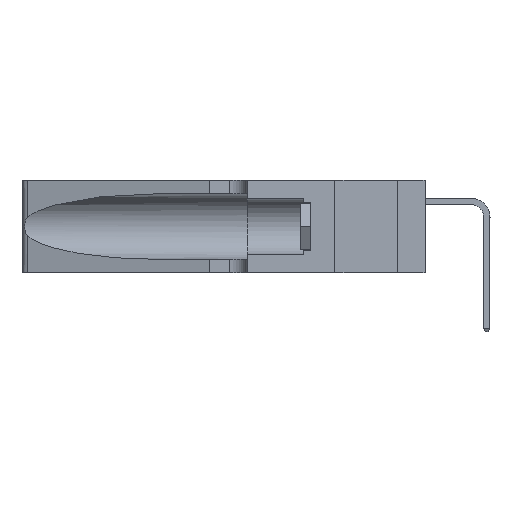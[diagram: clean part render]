
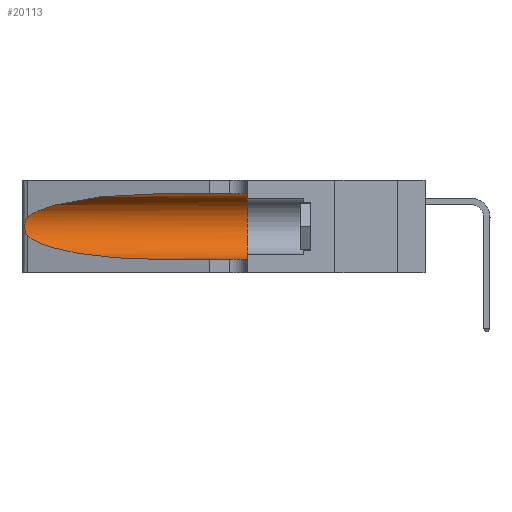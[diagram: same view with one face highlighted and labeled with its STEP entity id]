
A CAD part, left-side view. The second image highlights one B-rep face of the part: STEP entity #20113.
In plain terms, the highlighted cylindrical face has radius 3.308 mm (diameter 6.617 mm), a partial arc.
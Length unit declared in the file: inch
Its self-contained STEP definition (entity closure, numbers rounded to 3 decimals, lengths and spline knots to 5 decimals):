
#367 = B_SPLINE_CURVE_WITH_KNOTS ( 'NONE', 3,
 ( #2973, #14654, #8839, #22575, #10785, #24509, #12739, #1071, #14736, #3061, #16752, #5017, #18703, #6977 ),
 .UNSPECIFIED., .F., .F.,
 ( 4, 2, 2, 2, 2, 2, 4 ),
 ( 0., 0.00027, 0.00053, 0.00107, 0.0016, 0.00187, 0.00214 ),
 .UNSPECIFIED. ) ;
#808 = CARTESIAN_POINT ( 'NONE',  ( 0.25487, 1.22718, 0.14631 ) ) ;
#1071 = CARTESIAN_POINT ( 'NONE',  ( 0.26075, 1.23896, 0.178 ) ) ;
#1658 = VERTEX_POINT ( 'NONE', #12820 ) ;
#1889 = EDGE_CURVE ( 'NONE', #17701, #10730, #15651, .T. ) ;
#2789 = CARTESIAN_POINT ( 'NONE',  ( 0.1305, 0.72297, 0.31525 ) ) ;
#2973 = CARTESIAN_POINT ( 'NONE',  ( 0.25487, 1.22718, 0.22369 ) ) ;
#3061 = CARTESIAN_POINT ( 'NONE',  ( 0.25856, 1.23593, 0.16098 ) ) ;
#3597 = AXIS2_PLACEMENT_3D ( 'NONE', #19043, #22995, #11213 ) ;
#3985 = DIRECTION ( 'NONE',  ( 0., -1., 0. ) ) ;
#4210 = ORIENTED_EDGE ( 'NONE', *, *, #18114, .T. ) ;
#4444 = VECTOR ( 'NONE', #5754, 39.37008 ) ;
#4894 = EDGE_CURVE ( 'NONE', #23145, #14350, #22512, .T. ) ;
#5017 = CARTESIAN_POINT ( 'NONE',  ( 0.25639, 1.23186, 0.15144 ) ) ;
#5339 = VERTEX_POINT ( 'NONE', #7883 ) ;
#5754 = DIRECTION ( 'NONE',  ( 0., -1., 0. ) ) ;
#5861 = DIRECTION ( 'NONE',  ( 0., 1., 0. ) ) ;
#5895 = ORIENTED_EDGE ( 'NONE', *, *, #16063, .F. ) ;
#6423 = CARTESIAN_POINT ( 'NONE',  ( 0.1305, 0.72297, 0.05475 ) ) ;
#6775 = CARTESIAN_POINT ( 'NONE',  ( 0.1305, 0.35, 0.05475 ) ) ;
#6977 = CARTESIAN_POINT ( 'NONE',  ( 0.25487, 1.22718, 0.14631 ) ) ;
#7883 = CARTESIAN_POINT ( 'NONE',  ( 0.25487, 1.22718, 0.22369 ) ) ;
#8573 = CARTESIAN_POINT ( 'NONE',  ( 0.2373, 1.15595, 0.08982 ) ) ;
#8663 = CARTESIAN_POINT ( 'NONE',  ( 0.2373, 1.15595, 0.28018 ) ) ;
#8712 = CARTESIAN_POINT ( 'NONE',  ( 0.1305, 0.35, 0.31525 ) ) ;
#8839 = CARTESIAN_POINT ( 'NONE',  ( 0.25639, 1.23184, 0.21858 ) ) ;
#9137 = LINE ( 'NONE', #19554, #23550 ) ;
#10332 = CARTESIAN_POINT ( 'NONE',  ( 0.25487, 1.22718, 0.14631 ) ) ;
#10730 = VERTEX_POINT ( 'NONE', #6775 ) ;
#10785 = CARTESIAN_POINT ( 'NONE',  ( 0.25854, 1.2359, 0.20912 ) ) ;
#11213 = DIRECTION ( 'NONE',  ( 0., 0., -1. ) ) ;
#12739 = CARTESIAN_POINT ( 'NONE',  ( 0.26075, 1.23896, 0.19203 ) ) ;
#12820 = CARTESIAN_POINT ( 'NONE',  ( 0.1305, 0.72297, 0.31525 ) ) ;
#13416 = FACE_OUTER_BOUND ( 'NONE', #20971, .T. ) ;
#13856 = ORIENTED_EDGE ( 'NONE', *, *, #25141, .T. ) ;
#14350 = VERTEX_POINT ( 'NONE', #6423 ) ;
#14469 = CARTESIAN_POINT ( 'NONE',  ( 0.1305, 0.72297, 0.05475 ) ) ;
#14475 = CARTESIAN_POINT ( 'NONE',  ( 0.18966, 0.96281, 0.31525 ) ) ;
#14654 = CARTESIAN_POINT ( 'NONE',  ( 0.25555, 1.22994, 0.2215 ) ) ;
#14736 = CARTESIAN_POINT ( 'NONE',  ( 0.26017, 1.23833, 0.17102 ) ) ;
#15651 = CIRCLE ( 'NONE', #23735, 0.13025 ) ;
#15789 =( BOUNDED_CURVE ( )  B_SPLINE_CURVE ( 3, ( #2789, #14475, #8663, #22404 ),
 .UNSPECIFIED., .F., .T. ) 
 B_SPLINE_CURVE_WITH_KNOTS ( ( 4, 4 ),
 ( 1.5708, 2.84003 ),
 .UNSPECIFIED. ) 
 CURVE ( )  GEOMETRIC_REPRESENTATION_ITEM ( )  RATIONAL_B_SPLINE_CURVE ( ( 1., 0.87, 0.87, 1. ) ) 
 REPRESENTATION_ITEM ( '' )  );
#16063 = EDGE_CURVE ( 'NONE', #1658, #17701, #20070, .T. ) ;
#16752 = CARTESIAN_POINT ( 'NONE',  ( 0.25789, 1.23486, 0.15765 ) ) ;
#17056 = ORIENTED_EDGE ( 'NONE', *, *, #4894, .T. ) ;
#17568 = CARTESIAN_POINT ( 'NONE',  ( 0.1305, 0.35, 0.185 ) ) ;
#17701 = VERTEX_POINT ( 'NONE', #8712 ) ;
#18016 = ORIENTED_EDGE ( 'NONE', *, *, #20308, .T. ) ;
#18114 = EDGE_CURVE ( 'NONE', #5339, #23145, #367, .T. ) ;
#18703 = CARTESIAN_POINT ( 'NONE',  ( 0.25555, 1.22993, 0.14849 ) ) ;
#19043 = CARTESIAN_POINT ( 'NONE',  ( 0.1305, 1.61858, 0.185 ) ) ;
#19443 = CARTESIAN_POINT ( 'NONE',  ( 0.1305, 1.61858, 0.31525 ) ) ;
#19544 = DIRECTION ( 'NONE',  ( 0., 0., 1. ) ) ;
#19554 = CARTESIAN_POINT ( 'NONE',  ( 0.1305, 1.61858, 0.05475 ) ) ;
#20070 = LINE ( 'NONE', #19443, #4444 ) ;
#20113 = ADVANCED_FACE ( 'NONE', ( #13416 ), #23269, .F. ) ;
#20308 = EDGE_CURVE ( 'NONE', #14350, #10730, #9137, .T. ) ;
#20347 = CARTESIAN_POINT ( 'NONE',  ( 0.18966, 0.96281, 0.05475 ) ) ;
#20971 = EDGE_LOOP ( 'NONE', ( #13856, #4210, #17056, #18016, #22084, #5895 ) ) ;
#22084 = ORIENTED_EDGE ( 'NONE', *, *, #1889, .F. ) ;
#22404 = CARTESIAN_POINT ( 'NONE',  ( 0.25487, 1.22718, 0.22369 ) ) ;
#22512 =( BOUNDED_CURVE ( )  B_SPLINE_CURVE ( 3, ( #808, #8573, #20347, #14469 ),
 .UNSPECIFIED., .F., .F. ) 
 B_SPLINE_CURVE_WITH_KNOTS ( ( 4, 4 ),
 ( 3.44316, 4.71239 ),
 .UNSPECIFIED. ) 
 CURVE ( )  GEOMETRIC_REPRESENTATION_ITEM ( )  RATIONAL_B_SPLINE_CURVE ( ( 1., 0.87, 0.87, 1. ) ) 
 REPRESENTATION_ITEM ( '' )  );
#22575 = CARTESIAN_POINT ( 'NONE',  ( 0.25787, 1.23484, 0.2124 ) ) ;
#22995 = DIRECTION ( 'NONE',  ( 0., -1., 0. ) ) ;
#23145 = VERTEX_POINT ( 'NONE', #10332 ) ;
#23269 = CYLINDRICAL_SURFACE ( 'NONE', #3597, 0.13025 ) ;
#23550 = VECTOR ( 'NONE', #3985, 39.37008 ) ;
#23735 = AXIS2_PLACEMENT_3D ( 'NONE', #17568, #5861, #19544 ) ;
#24509 = CARTESIAN_POINT ( 'NONE',  ( 0.26018, 1.23835, 0.19895 ) ) ;
#25141 = EDGE_CURVE ( 'NONE', #1658, #5339, #15789, .T. ) ;
